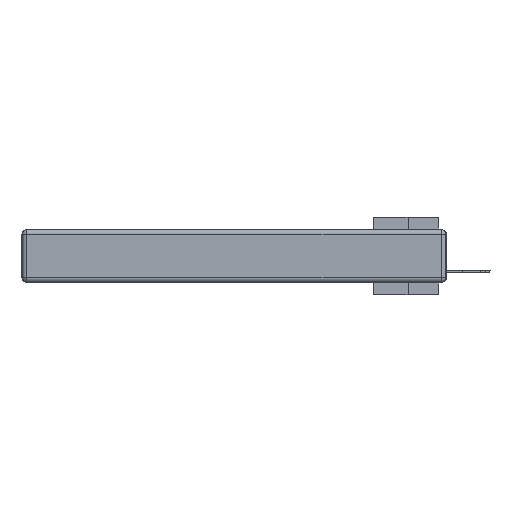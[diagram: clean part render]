
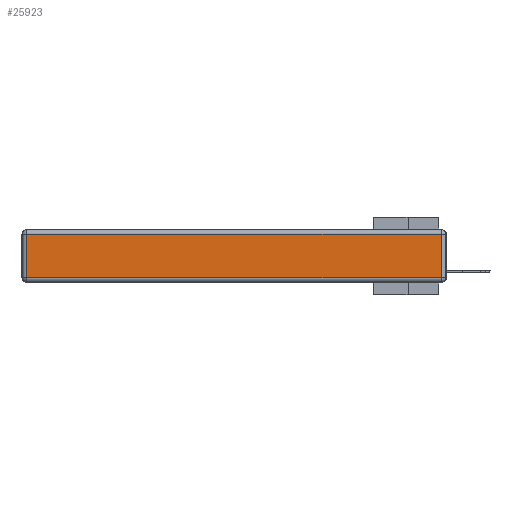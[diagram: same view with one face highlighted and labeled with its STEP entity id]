
A CAD part, left-side view. The second image highlights one B-rep face of the part: STEP entity #25923.
In plain terms, the highlighted planar face has unit normal (-1, 0, 0).
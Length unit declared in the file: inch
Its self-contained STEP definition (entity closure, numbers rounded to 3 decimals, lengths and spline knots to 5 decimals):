
#747 = CARTESIAN_POINT ( 'NONE',  ( 0., 2.72, -0.03 ) ) ;
#2157 = VECTOR ( 'NONE', #21853, 39.37008 ) ;
#2782 = CARTESIAN_POINT ( 'NONE',  ( 0., 2.75, -0.03 ) ) ;
#4425 = DIRECTION ( 'NONE',  ( 0., 0., 1. ) ) ;
#4782 = CARTESIAN_POINT ( 'NONE',  ( 0., 2.72, -0.313 ) ) ;
#4822 = VERTEX_POINT ( 'NONE', #4782 ) ;
#5027 = AXIS2_PLACEMENT_3D ( 'NONE', #28241, #30500, #4425 ) ;
#6375 = VECTOR ( 'NONE', #10760, 39.37008 ) ;
#6934 = CARTESIAN_POINT ( 'NONE',  ( 0., 2.72, -0.343 ) ) ;
#7027 = FACE_OUTER_BOUND ( 'NONE', #32274, .T. ) ;
#7127 = LINE ( 'NONE', #6934, #10946 ) ;
#10464 = EDGE_CURVE ( 'NONE', #28769, #4822, #7127, .T. ) ;
#10760 = DIRECTION ( 'NONE',  ( 0., 1., 0. ) ) ;
#10946 = VECTOR ( 'NONE', #22917, 39.37008 ) ;
#11210 = EDGE_CURVE ( 'NONE', #12441, #21290, #30334, .T. ) ;
#11483 = ORIENTED_EDGE ( 'NONE', *, *, #11210, .T. ) ;
#11611 = LINE ( 'NONE', #27393, #2157 ) ;
#11840 = ORIENTED_EDGE ( 'NONE', *, *, #24035, .T. ) ;
#12441 = VERTEX_POINT ( 'NONE', #14535 ) ;
#14535 = CARTESIAN_POINT ( 'NONE',  ( 0., 0.03, -0.313 ) ) ;
#17644 = PLANE ( 'NONE',  #5027 ) ;
#19261 = LINE ( 'NONE', #2782, #6375 ) ;
#21290 = VERTEX_POINT ( 'NONE', #27662 ) ;
#21853 = DIRECTION ( 'NONE',  ( 0., -1., 0. ) ) ;
#22917 = DIRECTION ( 'NONE',  ( 0., 0., -1. ) ) ;
#24035 = EDGE_CURVE ( 'NONE', #4822, #12441, #11611, .T. ) ;
#24422 = DIRECTION ( 'NONE',  ( 0., 0., 1. ) ) ;
#25923 = ADVANCED_FACE ( 'NONE', ( #7027 ), #17644, .T. ) ;
#27393 = CARTESIAN_POINT ( 'NONE',  ( 0., 0., -0.313 ) ) ;
#27662 = CARTESIAN_POINT ( 'NONE',  ( 0., 0.03, -0.03 ) ) ;
#27828 = ORIENTED_EDGE ( 'NONE', *, *, #31713, .T. ) ;
#28241 = CARTESIAN_POINT ( 'NONE',  ( 0., 0., -0.343 ) ) ;
#28769 = VERTEX_POINT ( 'NONE', #747 ) ;
#30334 = LINE ( 'NONE', #30510, #31982 ) ;
#30500 = DIRECTION ( 'NONE',  ( -1., 0., 0. ) ) ;
#30510 = CARTESIAN_POINT ( 'NONE',  ( 0., 0.03, -0.343 ) ) ;
#31713 = EDGE_CURVE ( 'NONE', #21290, #28769, #19261, .T. ) ;
#31982 = VECTOR ( 'NONE', #24422, 39.37008 ) ;
#32274 = EDGE_LOOP ( 'NONE', ( #11840, #11483, #27828, #34097 ) ) ;
#34097 = ORIENTED_EDGE ( 'NONE', *, *, #10464, .T. ) ;
